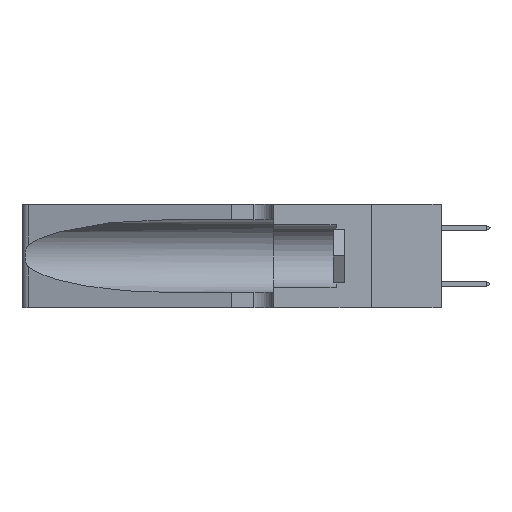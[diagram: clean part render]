
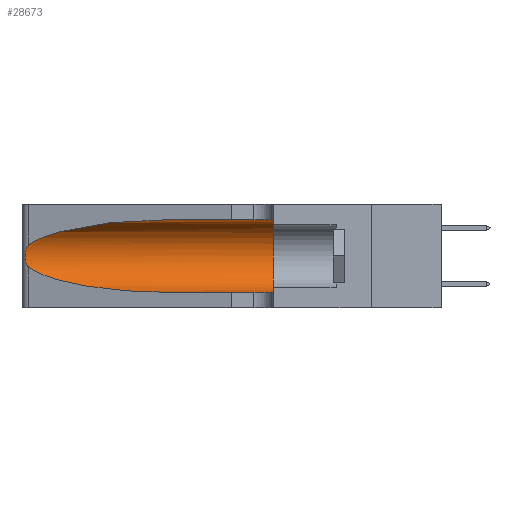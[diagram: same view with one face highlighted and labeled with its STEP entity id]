
A CAD part, left-side view. The second image highlights one B-rep face of the part: STEP entity #28673.
In plain terms, the highlighted cylindrical face has radius 3.308 mm (diameter 6.617 mm), a partial arc.
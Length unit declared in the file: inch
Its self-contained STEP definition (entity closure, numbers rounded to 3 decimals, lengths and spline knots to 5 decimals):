
#320 = LINE ( 'NONE', #9919, #5905 ) ;
#1921 = CARTESIAN_POINT ( 'NONE',  ( 0.25487, 1.22718, 0.22369 ) ) ;
#2570 = ORIENTED_EDGE ( 'NONE', *, *, #26538, .T. ) ;
#3763 = VERTEX_POINT ( 'NONE', #18713 ) ;
#3852 = CARTESIAN_POINT ( 'NONE',  ( 0.25487, 1.22718, 0.22369 ) ) ;
#4843 = VERTEX_POINT ( 'NONE', #26881 ) ;
#5561 = CARTESIAN_POINT ( 'NONE',  ( 0.1305, 1.61858, 0.05475 ) ) ;
#5905 = VECTOR ( 'NONE', #29123, 39.37008 ) ;
#6513 = CARTESIAN_POINT ( 'NONE',  ( 0.18966, 0.96281, 0.05475 ) ) ;
#6694 = CARTESIAN_POINT ( 'NONE',  ( 0.26018, 1.23835, 0.19895 ) ) ;
#7220 = VERTEX_POINT ( 'NONE', #18758 ) ;
#8491 = CARTESIAN_POINT ( 'NONE',  ( 0.18966, 0.96281, 0.31525 ) ) ;
#8897 = AXIS2_PLACEMENT_3D ( 'NONE', #36475, #18127, #10222 ) ;
#9766 = CARTESIAN_POINT ( 'NONE',  ( 0.25487, 1.22718, 0.22369 ) ) ;
#9897 = CARTESIAN_POINT ( 'NONE',  ( 0.25639, 1.23186, 0.15144 ) ) ;
#9919 = CARTESIAN_POINT ( 'NONE',  ( 0.1305, 1.61858, 0.31525 ) ) ;
#10222 = DIRECTION ( 'NONE',  ( 0., 0., 1. ) ) ;
#10289 = EDGE_LOOP ( 'NONE', ( #22484, #36980, #2570, #15843, #21141, #17875 ) ) ;
#11263 = CIRCLE ( 'NONE', #8897, 0.13025 ) ;
#11636 =( BOUNDED_CURVE ( )  B_SPLINE_CURVE ( 3, ( #13317, #8491, #13415, #3852 ),
 .UNSPECIFIED., .F., .T. ) 
 B_SPLINE_CURVE_WITH_KNOTS ( ( 4, 4 ),
 ( 1.5708, 2.84003 ),
 .UNSPECIFIED. ) 
 CURVE ( )  GEOMETRIC_REPRESENTATION_ITEM ( )  RATIONAL_B_SPLINE_CURVE ( ( 1., 0.87, 0.87, 1. ) ) 
 REPRESENTATION_ITEM ( '' )  );
#13283 = CARTESIAN_POINT ( 'NONE',  ( 0.25487, 1.22718, 0.14631 ) ) ;
#13317 = CARTESIAN_POINT ( 'NONE',  ( 0.1305, 0.72297, 0.31525 ) ) ;
#13415 = CARTESIAN_POINT ( 'NONE',  ( 0.2373, 1.15595, 0.28018 ) ) ;
#14032 = EDGE_CURVE ( 'NONE', #7220, #4843, #11263, .T. ) ;
#15361 = CYLINDRICAL_SURFACE ( 'NONE', #32836, 0.13025 ) ;
#15843 = ORIENTED_EDGE ( 'NONE', *, *, #18868, .T. ) ;
#16018 = CARTESIAN_POINT ( 'NONE',  ( 0.25555, 1.22993, 0.14849 ) ) ;
#16231 = CARTESIAN_POINT ( 'NONE',  ( 0.1305, 0.72297, 0.05475 ) ) ;
#16478 = VERTEX_POINT ( 'NONE', #33451 ) ;
#17520 = EDGE_CURVE ( 'NONE', #3763, #22222, #11636, .T. ) ;
#17875 = ORIENTED_EDGE ( 'NONE', *, *, #37384, .F. ) ;
#18127 = DIRECTION ( 'NONE',  ( 0., 1., 0. ) ) ;
#18493 = DIRECTION ( 'NONE',  ( 0., -1., 0. ) ) ;
#18713 = CARTESIAN_POINT ( 'NONE',  ( 0.1305, 0.72297, 0.31525 ) ) ;
#18758 = CARTESIAN_POINT ( 'NONE',  ( 0.1305, 0.35, 0.31525 ) ) ;
#18868 = EDGE_CURVE ( 'NONE', #16478, #4843, #41664, .T. ) ;
#19219 = CARTESIAN_POINT ( 'NONE',  ( 0.25639, 1.23184, 0.21858 ) ) ;
#19299 = CARTESIAN_POINT ( 'NONE',  ( 0.2373, 1.15595, 0.08982 ) ) ;
#20606 =( BOUNDED_CURVE ( )  B_SPLINE_CURVE ( 3, ( #22573, #19299, #6513, #16231 ),
 .UNSPECIFIED., .F., .F. ) 
 B_SPLINE_CURVE_WITH_KNOTS ( ( 4, 4 ),
 ( 3.44316, 4.71239 ),
 .UNSPECIFIED. ) 
 CURVE ( )  GEOMETRIC_REPRESENTATION_ITEM ( )  RATIONAL_B_SPLINE_CURVE ( ( 1., 0.87, 0.87, 1. ) ) 
 REPRESENTATION_ITEM ( '' )  );
#21141 = ORIENTED_EDGE ( 'NONE', *, *, #14032, .F. ) ;
#22222 = VERTEX_POINT ( 'NONE', #1921 ) ;
#22484 = ORIENTED_EDGE ( 'NONE', *, *, #17520, .T. ) ;
#22573 = CARTESIAN_POINT ( 'NONE',  ( 0.25487, 1.22718, 0.14631 ) ) ;
#22753 = CARTESIAN_POINT ( 'NONE',  ( 0.26017, 1.23833, 0.17102 ) ) ;
#22888 = CARTESIAN_POINT ( 'NONE',  ( 0.25789, 1.23486, 0.15765 ) ) ;
#22979 = VECTOR ( 'NONE', #18493, 39.37008 ) ;
#23027 = CARTESIAN_POINT ( 'NONE',  ( 0.25555, 1.22994, 0.2215 ) ) ;
#23641 = CARTESIAN_POINT ( 'NONE',  ( 0.25854, 1.2359, 0.20912 ) ) ;
#26277 = CARTESIAN_POINT ( 'NONE',  ( 0.26075, 1.23896, 0.19203 ) ) ;
#26538 = EDGE_CURVE ( 'NONE', #39844, #16478, #20606, .T. ) ;
#26881 = CARTESIAN_POINT ( 'NONE',  ( 0.1305, 0.35, 0.05475 ) ) ;
#27465 = DIRECTION ( 'NONE',  ( 0., 0., -1. ) ) ;
#27747 = DIRECTION ( 'NONE',  ( 0., -1., 0. ) ) ;
#28673 = ADVANCED_FACE ( 'NONE', ( #34545 ), #15361, .F. ) ;
#29123 = DIRECTION ( 'NONE',  ( 0., -1., 0. ) ) ;
#29239 = CARTESIAN_POINT ( 'NONE',  ( 0.26075, 1.23896, 0.178 ) ) ;
#30948 = EDGE_CURVE ( 'NONE', #22222, #39844, #37468, .T. ) ;
#32317 = CARTESIAN_POINT ( 'NONE',  ( 0.25487, 1.22718, 0.14631 ) ) ;
#32836 = AXIS2_PLACEMENT_3D ( 'NONE', #34104, #27747, #27465 ) ;
#33451 = CARTESIAN_POINT ( 'NONE',  ( 0.1305, 0.72297, 0.05475 ) ) ;
#34104 = CARTESIAN_POINT ( 'NONE',  ( 0.1305, 1.61858, 0.185 ) ) ;
#34545 = FACE_OUTER_BOUND ( 'NONE', #10289, .T. ) ;
#36475 = CARTESIAN_POINT ( 'NONE',  ( 0.1305, 0.35, 0.185 ) ) ;
#36980 = ORIENTED_EDGE ( 'NONE', *, *, #30948, .T. ) ;
#37384 = EDGE_CURVE ( 'NONE', #3763, #7220, #320, .T. ) ;
#37468 = B_SPLINE_CURVE_WITH_KNOTS ( 'NONE', 3,
 ( #9766, #23027, #19219, #39090, #23641, #6694, #26277, #29239, #22753, #38964, #22888, #9897, #16018, #32317 ),
 .UNSPECIFIED., .F., .F.,
 ( 4, 2, 2, 2, 2, 2, 4 ),
 ( 0., 0.00027, 0.00053, 0.00107, 0.0016, 0.00187, 0.00214 ),
 .UNSPECIFIED. ) ;
#38964 = CARTESIAN_POINT ( 'NONE',  ( 0.25856, 1.23593, 0.16098 ) ) ;
#39090 = CARTESIAN_POINT ( 'NONE',  ( 0.25787, 1.23484, 0.2124 ) ) ;
#39844 = VERTEX_POINT ( 'NONE', #13283 ) ;
#41664 = LINE ( 'NONE', #5561, #22979 ) ;
